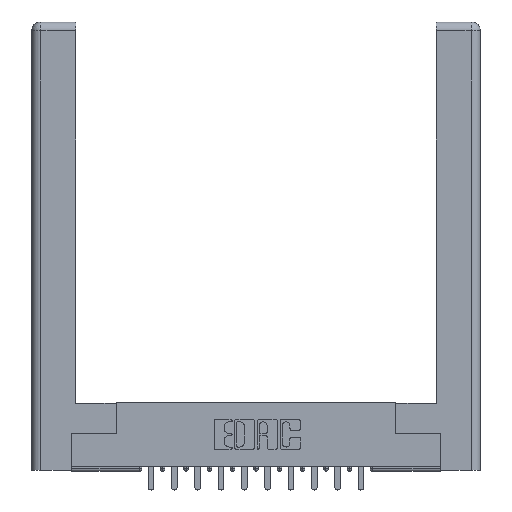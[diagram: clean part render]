
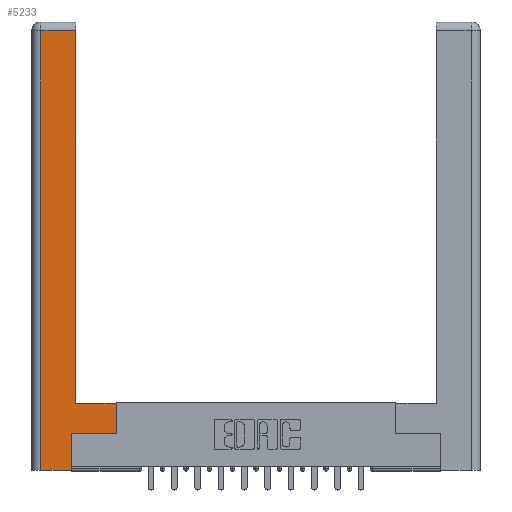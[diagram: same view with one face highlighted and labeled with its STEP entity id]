
A CAD part, top view. The second image highlights one B-rep face of the part: STEP entity #5233.
In plain terms, the highlighted planar face has unit normal (0, 0, 1).
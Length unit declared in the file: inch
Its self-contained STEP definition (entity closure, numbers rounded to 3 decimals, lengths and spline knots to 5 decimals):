
#250 = LINE ( 'NONE', #11401, #12946 ) ;
#257 = EDGE_CURVE ( 'NONE', #6960, #9894, #3720, .T. ) ;
#905 = CARTESIAN_POINT ( 'NONE',  ( 0.565, 0.245, 0. ) ) ;
#1129 = DIRECTION ( 'NONE',  ( 1., 0., 0. ) ) ;
#1330 = LINE ( 'NONE', #3911, #5527 ) ;
#1335 = FACE_OUTER_BOUND ( 'NONE', #4374, .T. ) ;
#1542 = ORIENTED_EDGE ( 'NONE', *, *, #14357, .T. ) ;
#1829 = VECTOR ( 'NONE', #14943, 39.37008 ) ;
#1956 = VERTEX_POINT ( 'NONE', #9946 ) ;
#2730 = DIRECTION ( 'NONE',  ( 0., 1., 0. ) ) ;
#2909 = ORIENTED_EDGE ( 'NONE', *, *, #10044, .T. ) ;
#3182 = CARTESIAN_POINT ( 'NONE',  ( 0.265, 0., 0. ) ) ;
#3214 = CARTESIAN_POINT ( 'NONE',  ( 0.265, 0.245, 0. ) ) ;
#3554 = CARTESIAN_POINT ( 'NONE',  ( 0.295, 3., 0. ) ) ;
#3720 = LINE ( 'NONE', #12275, #1829 ) ;
#3739 = VERTEX_POINT ( 'NONE', #6977 ) ;
#3828 = DIRECTION ( 'NONE',  ( 0., 0., -1. ) ) ;
#3911 = CARTESIAN_POINT ( 'NONE',  ( 0.0615, 0., 0. ) ) ;
#3915 = PLANE ( 'NONE',  #10133 ) ;
#4015 = EDGE_CURVE ( 'NONE', #3739, #14777, #1330, .T. ) ;
#4374 = EDGE_LOOP ( 'NONE', ( #14888, #2909, #15016, #10750, #6792, #12672, #1542, #11045 ) ) ;
#4485 = LINE ( 'NONE', #3182, #13258 ) ;
#4813 = DIRECTION ( 'NONE',  ( -1., 0., 0. ) ) ;
#5009 = LINE ( 'NONE', #12559, #16059 ) ;
#5204 = EDGE_CURVE ( 'NONE', #6020, #6960, #250, .T. ) ;
#5233 = ADVANCED_FACE ( 'NONE', ( #1335 ), #3915, .F. ) ;
#5527 = VECTOR ( 'NONE', #13837, 39.37008 ) ;
#6020 = VERTEX_POINT ( 'NONE', #13373 ) ;
#6486 = EDGE_CURVE ( 'NONE', #1956, #8281, #14686, .T. ) ;
#6792 = ORIENTED_EDGE ( 'NONE', *, *, #5204, .T. ) ;
#6960 = VERTEX_POINT ( 'NONE', #3214 ) ;
#6977 = CARTESIAN_POINT ( 'NONE',  ( 0.0615, 2.94, 0. ) ) ;
#7201 = LINE ( 'NONE', #8449, #9323 ) ;
#7310 = VERTEX_POINT ( 'NONE', #8525 ) ;
#7360 = EDGE_CURVE ( 'NONE', #7310, #1956, #7201, .T. ) ;
#7563 = DIRECTION ( 'NONE',  ( 0., 1., 0. ) ) ;
#8281 = VERTEX_POINT ( 'NONE', #13779 ) ;
#8449 = CARTESIAN_POINT ( 'NONE',  ( 0.295, 0.45, 0. ) ) ;
#8525 = CARTESIAN_POINT ( 'NONE',  ( 0.565, 0.45, 0. ) ) ;
#8997 = CARTESIAN_POINT ( 'NONE',  ( 0.565, 0.45, 0. ) ) ;
#9039 = DIRECTION ( 'NONE',  ( -1., 0., 0. ) ) ;
#9094 = VECTOR ( 'NONE', #12084, 39.37008 ) ;
#9323 = VECTOR ( 'NONE', #4813, 39.37008 ) ;
#9894 = VERTEX_POINT ( 'NONE', #905 ) ;
#9921 = DIRECTION ( 'NONE',  ( -1., 0., 0. ) ) ;
#9946 = CARTESIAN_POINT ( 'NONE',  ( 0.295, 0.45, 0. ) ) ;
#10044 = EDGE_CURVE ( 'NONE', #8281, #3739, #5009, .T. ) ;
#10133 = AXIS2_PLACEMENT_3D ( 'NONE', #13754, #3828, #9039 ) ;
#10750 = ORIENTED_EDGE ( 'NONE', *, *, #14882, .T. ) ;
#11045 = ORIENTED_EDGE ( 'NONE', *, *, #7360, .T. ) ;
#11401 = CARTESIAN_POINT ( 'NONE',  ( 0.265, 0.245, 0. ) ) ;
#12084 = DIRECTION ( 'NONE',  ( 0., 1., 0. ) ) ;
#12275 = CARTESIAN_POINT ( 'NONE',  ( 0.565, 0.245, 0. ) ) ;
#12559 = CARTESIAN_POINT ( 'NONE',  ( 0.0615, 2.94, 0. ) ) ;
#12639 = CARTESIAN_POINT ( 'NONE',  ( 0.0615, 0., 0. ) ) ;
#12672 = ORIENTED_EDGE ( 'NONE', *, *, #257, .T. ) ;
#12775 = VECTOR ( 'NONE', #2730, 39.37008 ) ;
#12946 = VECTOR ( 'NONE', #7563, 39.37008 ) ;
#13258 = VECTOR ( 'NONE', #1129, 39.37008 ) ;
#13373 = CARTESIAN_POINT ( 'NONE',  ( 0.265, 0., 0. ) ) ;
#13754 = CARTESIAN_POINT ( 'NONE',  ( 0., 0., 0. ) ) ;
#13779 = CARTESIAN_POINT ( 'NONE',  ( 0.295, 2.94, 0. ) ) ;
#13837 = DIRECTION ( 'NONE',  ( 0., -1., 0. ) ) ;
#14357 = EDGE_CURVE ( 'NONE', #9894, #7310, #15320, .T. ) ;
#14686 = LINE ( 'NONE', #3554, #9094 ) ;
#14777 = VERTEX_POINT ( 'NONE', #12639 ) ;
#14882 = EDGE_CURVE ( 'NONE', #14777, #6020, #4485, .T. ) ;
#14888 = ORIENTED_EDGE ( 'NONE', *, *, #6486, .T. ) ;
#14943 = DIRECTION ( 'NONE',  ( 1., 0., 0. ) ) ;
#15016 = ORIENTED_EDGE ( 'NONE', *, *, #4015, .T. ) ;
#15320 = LINE ( 'NONE', #8997, #12775 ) ;
#16059 = VECTOR ( 'NONE', #9921, 39.37008 ) ;
